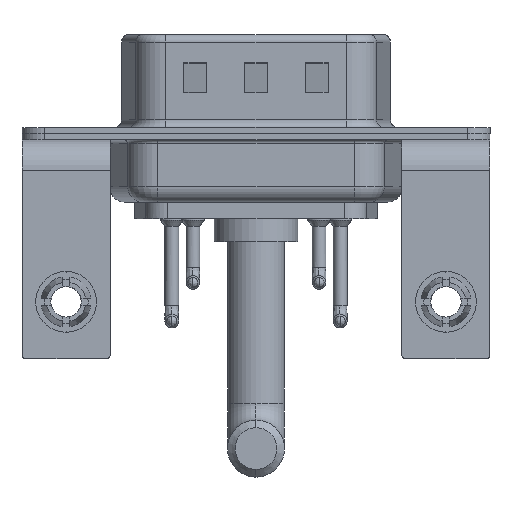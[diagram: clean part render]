
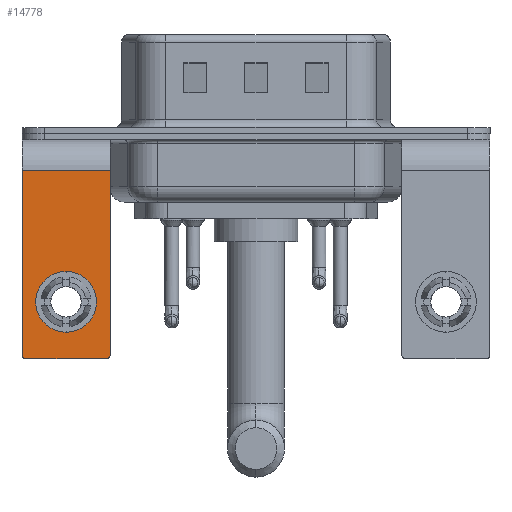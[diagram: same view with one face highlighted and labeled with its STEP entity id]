
A CAD part, front view. The second image highlights one B-rep face of the part: STEP entity #14778.
In plain terms, the highlighted planar face has unit normal (0, -1, 0).
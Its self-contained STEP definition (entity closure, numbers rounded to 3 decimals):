
#43 = ORIENTED_EDGE ( 'NONE', *, *, #11418, .F. ) ;
#57 = CARTESIAN_POINT ( 'NONE',  ( 0., -6.25, -9.07 ) ) ;
#392 = ORIENTED_EDGE ( 'NONE', *, *, #15326, .T. ) ;
#453 = CARTESIAN_POINT ( 'NONE',  ( 2.9, -6.25, -2.4 ) ) ;
#1317 = DIRECTION ( 'NONE',  ( 0., -1., 0. ) ) ;
#1435 = DIRECTION ( 'NONE',  ( 0., 0., -1. ) ) ;
#1579 = VECTOR ( 'NONE', #9061, 1000. ) ;
#1854 = ORIENTED_EDGE ( 'NONE', *, *, #4198, .T. ) ;
#1980 = DIRECTION ( 'NONE',  ( 0., -1., 0. ) ) ;
#2341 = LINE ( 'NONE', #8737, #1579 ) ;
#2730 = CARTESIAN_POINT ( 'NONE',  ( 2.9, -6.25, -14.55 ) ) ;
#3077 = CIRCLE ( 'NONE', #15372, 0.25 ) ;
#3604 = CARTESIAN_POINT ( 'NONE',  ( 0., -6.25, -13.07 ) ) ;
#4198 = EDGE_CURVE ( 'NONE', #10416, #17123, #15424, .T. ) ;
#4445 = VERTEX_POINT ( 'NONE', #3604 ) ;
#4533 = CARTESIAN_POINT ( 'NONE',  ( -2.9, -6.25, -2.4 ) ) ;
#4579 = EDGE_CURVE ( 'NONE', #16444, #4445, #15583, .T. ) ;
#5110 = VECTOR ( 'NONE', #18717, 1000. ) ;
#5336 = FACE_BOUND ( 'NONE', #6361, .T. ) ;
#5617 = DIRECTION ( 'NONE',  ( 0., 0., 1. ) ) ;
#5934 = AXIS2_PLACEMENT_3D ( 'NONE', #7799, #1317, #14498 ) ;
#6100 = AXIS2_PLACEMENT_3D ( 'NONE', #16363, #10841, #9300 ) ;
#6178 = CIRCLE ( 'NONE', #13894, 2. ) ;
#6361 = EDGE_LOOP ( 'NONE', ( #7986, #15398 ) ) ;
#7047 = VERTEX_POINT ( 'NONE', #10657 ) ;
#7136 = CARTESIAN_POINT ( 'NONE',  ( -2.65, -6.25, -14.8 ) ) ;
#7159 = AXIS2_PLACEMENT_3D ( 'NONE', #10279, #10511, #20408 ) ;
#7725 = ORIENTED_EDGE ( 'NONE', *, *, #16528, .F. ) ;
#7799 = CARTESIAN_POINT ( 'NONE',  ( 2.65, -6.25, -14.55 ) ) ;
#7986 = ORIENTED_EDGE ( 'NONE', *, *, #16800, .T. ) ;
#8682 = CARTESIAN_POINT ( 'NONE',  ( 2.65, -6.25, -14.8 ) ) ;
#8737 = CARTESIAN_POINT ( 'NONE',  ( 2.9, -6.25, -2.4 ) ) ;
#8864 = ORIENTED_EDGE ( 'NONE', *, *, #16964, .T. ) ;
#8884 = CARTESIAN_POINT ( 'NONE',  ( -2.9, -6.25, -2.4 ) ) ;
#9061 = DIRECTION ( 'NONE',  ( 0., 0., -1. ) ) ;
#9184 = VECTOR ( 'NONE', #17464, 1000. ) ;
#9300 = DIRECTION ( 'NONE',  ( 0., 0., 1. ) ) ;
#10279 = CARTESIAN_POINT ( 'NONE',  ( 2.9, -6.25, -2.4 ) ) ;
#10416 = VERTEX_POINT ( 'NONE', #8682 ) ;
#10511 = DIRECTION ( 'NONE',  ( 0., 1., 0. ) ) ;
#10657 = CARTESIAN_POINT ( 'NONE',  ( -2.9, -6.25, -14.55 ) ) ;
#10676 = VECTOR ( 'NONE', #1435, 1000. ) ;
#10841 = DIRECTION ( 'NONE',  ( 0., 1., 0. ) ) ;
#11418 = EDGE_CURVE ( 'NONE', #10416, #12684, #15496, .T. ) ;
#12143 = FACE_OUTER_BOUND ( 'NONE', #18111, .T. ) ;
#12217 = LINE ( 'NONE', #453, #5110 ) ;
#12684 = VERTEX_POINT ( 'NONE', #7136 ) ;
#12789 = DIRECTION ( 'NONE',  ( 0., 1., 0. ) ) ;
#13894 = AXIS2_PLACEMENT_3D ( 'NONE', #21139, #12789, #19506 ) ;
#14049 = CARTESIAN_POINT ( 'NONE',  ( 2.9, -6.25, -14.8 ) ) ;
#14078 = VERTEX_POINT ( 'NONE', #18680 ) ;
#14498 = DIRECTION ( 'NONE',  ( 0., 0., 1. ) ) ;
#14778 = ADVANCED_FACE ( 'NONE', ( #5336, #12143 ), #18875, .F. ) ;
#15326 = EDGE_CURVE ( 'NONE', #20473, #7047, #19586, .T. ) ;
#15372 = AXIS2_PLACEMENT_3D ( 'NONE', #20563, #1980, #5617 ) ;
#15398 = ORIENTED_EDGE ( 'NONE', *, *, #4579, .T. ) ;
#15424 = CIRCLE ( 'NONE', #5934, 0.25 ) ;
#15496 = LINE ( 'NONE', #14049, #9184 ) ;
#15583 = CIRCLE ( 'NONE', #6100, 2. ) ;
#15934 = ORIENTED_EDGE ( 'NONE', *, *, #20017, .T. ) ;
#16363 = CARTESIAN_POINT ( 'NONE',  ( 0., -6.25, -11.07 ) ) ;
#16444 = VERTEX_POINT ( 'NONE', #57 ) ;
#16528 = EDGE_CURVE ( 'NONE', #14078, #17123, #2341, .T. ) ;
#16800 = EDGE_CURVE ( 'NONE', #4445, #16444, #6178, .T. ) ;
#16964 = EDGE_CURVE ( 'NONE', #14078, #20473, #12217, .T. ) ;
#17123 = VERTEX_POINT ( 'NONE', #2730 ) ;
#17464 = DIRECTION ( 'NONE',  ( -1., 0., 0. ) ) ;
#18111 = EDGE_LOOP ( 'NONE', ( #392, #15934, #43, #1854, #7725, #8864 ) ) ;
#18680 = CARTESIAN_POINT ( 'NONE',  ( 2.9, -6.25, -2.4 ) ) ;
#18717 = DIRECTION ( 'NONE',  ( -1., 0., 0. ) ) ;
#18875 = PLANE ( 'NONE',  #7159 ) ;
#19506 = DIRECTION ( 'NONE',  ( 0., 0., 1. ) ) ;
#19586 = LINE ( 'NONE', #4533, #10676 ) ;
#20017 = EDGE_CURVE ( 'NONE', #7047, #12684, #3077, .T. ) ;
#20408 = DIRECTION ( 'NONE',  ( 0., 0., 1. ) ) ;
#20473 = VERTEX_POINT ( 'NONE', #8884 ) ;
#20563 = CARTESIAN_POINT ( 'NONE',  ( -2.65, -6.25, -14.55 ) ) ;
#21139 = CARTESIAN_POINT ( 'NONE',  ( 0., -6.25, -11.07 ) ) ;
